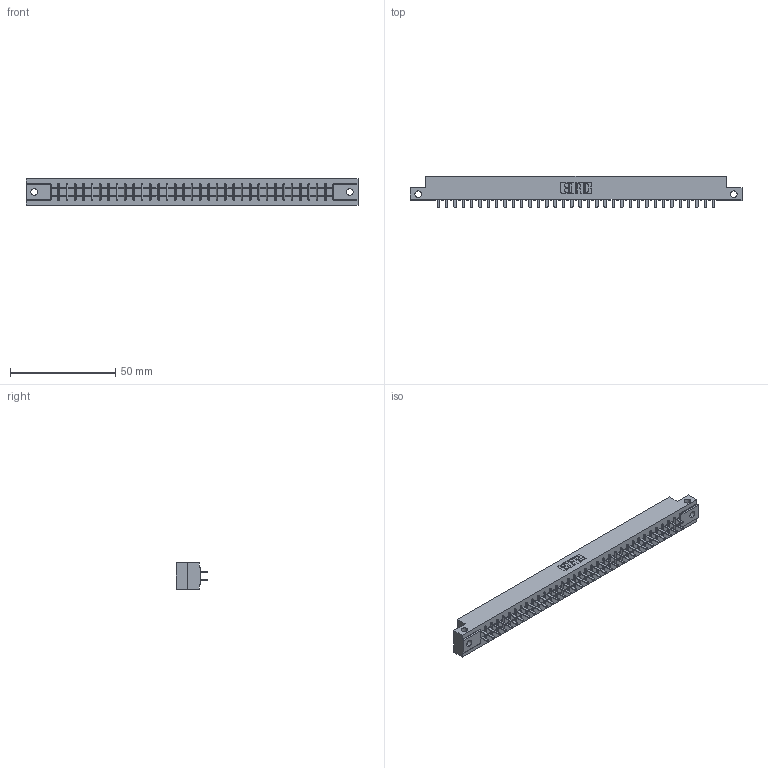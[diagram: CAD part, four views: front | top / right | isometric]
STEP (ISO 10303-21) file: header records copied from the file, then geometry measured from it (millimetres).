
FILE_DESCRIPTION (( 'STEP AP203' ), '1' );
FILE_NAME ('315-068-521-212.STEP', '2020-09-20T03:45:59', ( '' ), ( '' ), 'SwSTEP 2.0', 'SolidWorks 2020', '' );
FILE_SCHEMA (( 'CONFIG_CONTROL_DESIGN' ));
Length unit declared in the file: inch
Products named in the file (3): 315-068-521-212; 305 Part_.128 Dia; 305-290-001_521
Assembly tree (69 placements, depth 2):
  315-068-521-212
    305 Part_.128 Dia
    305-290-001_521  x68
Bounding box: 157.73 x 14.86 x 12.7 mm (x, y, z)
Volume: 16145.5 mm3; surface area: 20107.9 mm2
Topology: 69 solids, 69 shells, 3256 faces, 9294 edges, 6008 vertices
Faces by surface type: plane 1904, cylinder 1216, sphere 136
Entity records: 38073 total; most frequent: CARTESIAN_POINT 6348, ORIENTED_EDGE 6256, DIRECTION 6086, EDGE_CURVE 3128, LINE 2506, VECTOR 2506, VERTEX_POINT 1988, AXIS2_PLACEMENT_3D 1790
